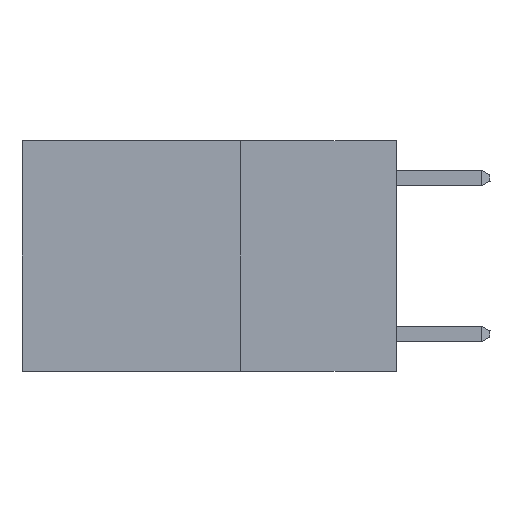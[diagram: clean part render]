
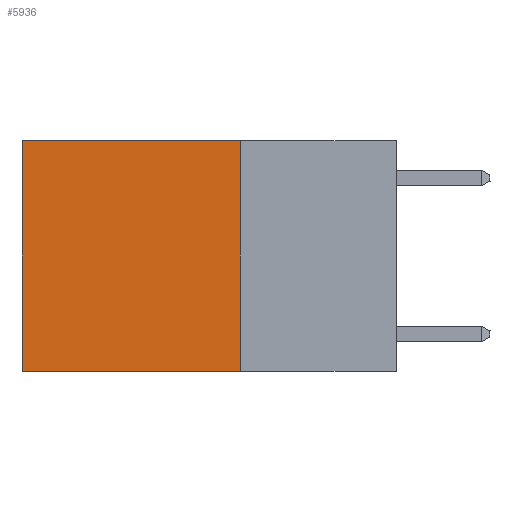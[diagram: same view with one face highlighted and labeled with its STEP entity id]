
A CAD part, left-side view. The second image highlights one B-rep face of the part: STEP entity #5936.
In plain terms, the highlighted planar face has unit normal (-1, 0, 0).
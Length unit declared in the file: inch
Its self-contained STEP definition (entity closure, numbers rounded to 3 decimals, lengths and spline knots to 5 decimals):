
#348 = VECTOR ( 'NONE', #10414, 39.37008 ) ;
#420 = DIRECTION ( 'NONE',  ( 1., 0., 0. ) ) ;
#1305 = VECTOR ( 'NONE', #6958, 39.37008 ) ;
#1930 = CARTESIAN_POINT ( 'NONE',  ( 0.2625, 0.25, -0.37 ) ) ;
#2312 = LINE ( 'NONE', #11854, #11829 ) ;
#2341 = AXIS2_PLACEMENT_3D ( 'NONE', #9613, #420, #6902 ) ;
#2505 = CARTESIAN_POINT ( 'NONE',  ( 0.2625, 0.6, 0. ) ) ;
#2656 = EDGE_CURVE ( 'NONE', #2916, #10417, #11467, .T. ) ;
#2916 = VERTEX_POINT ( 'NONE', #5875 ) ;
#3062 = CARTESIAN_POINT ( 'NONE',  ( 0.2625, 0.6, 0. ) ) ;
#4618 = FACE_OUTER_BOUND ( 'NONE', #4995, .T. ) ;
#4690 = CARTESIAN_POINT ( 'NONE',  ( 0.2625, 0.25, 0. ) ) ;
#4995 = EDGE_LOOP ( 'NONE', ( #5566, #7248, #6139, #5982 ) ) ;
#5560 = EDGE_CURVE ( 'NONE', #10417, #6856, #2312, .T. ) ;
#5566 = ORIENTED_EDGE ( 'NONE', *, *, #5903, .T. ) ;
#5586 = CARTESIAN_POINT ( 'NONE',  ( 0.2625, 0.6, -0.37 ) ) ;
#5875 = CARTESIAN_POINT ( 'NONE',  ( 0.2625, 0.25, 0. ) ) ;
#5903 = EDGE_CURVE ( 'NONE', #11801, #6856, #7198, .T. ) ;
#5936 = ADVANCED_FACE ( 'NONE', ( #4618 ), #7711, .F. ) ;
#5982 = ORIENTED_EDGE ( 'NONE', *, *, #11264, .T. ) ;
#6139 = ORIENTED_EDGE ( 'NONE', *, *, #2656, .F. ) ;
#6495 = DIRECTION ( 'NONE',  ( 0., 1., 0. ) ) ;
#6856 = VERTEX_POINT ( 'NONE', #5586 ) ;
#6902 = DIRECTION ( 'NONE',  ( 0., 0., -1. ) ) ;
#6958 = DIRECTION ( 'NONE',  ( 0., 0., -1. ) ) ;
#7198 = LINE ( 'NONE', #2505, #1305 ) ;
#7248 = ORIENTED_EDGE ( 'NONE', *, *, #5560, .F. ) ;
#7711 = PLANE ( 'NONE',  #2341 ) ;
#7898 = LINE ( 'NONE', #7983, #10089 ) ;
#7983 = CARTESIAN_POINT ( 'NONE',  ( 0.2625, 0.25, 0. ) ) ;
#8061 = DIRECTION ( 'NONE',  ( 0., 1., 0. ) ) ;
#9613 = CARTESIAN_POINT ( 'NONE',  ( 0.2625, 0.25, 0. ) ) ;
#10089 = VECTOR ( 'NONE', #8061, 39.37008 ) ;
#10414 = DIRECTION ( 'NONE',  ( 0., 0., -1. ) ) ;
#10417 = VERTEX_POINT ( 'NONE', #1930 ) ;
#11264 = EDGE_CURVE ( 'NONE', #2916, #11801, #7898, .T. ) ;
#11467 = LINE ( 'NONE', #4690, #348 ) ;
#11801 = VERTEX_POINT ( 'NONE', #3062 ) ;
#11829 = VECTOR ( 'NONE', #6495, 39.37008 ) ;
#11854 = CARTESIAN_POINT ( 'NONE',  ( 0.2625, 0.25, -0.37 ) ) ;
